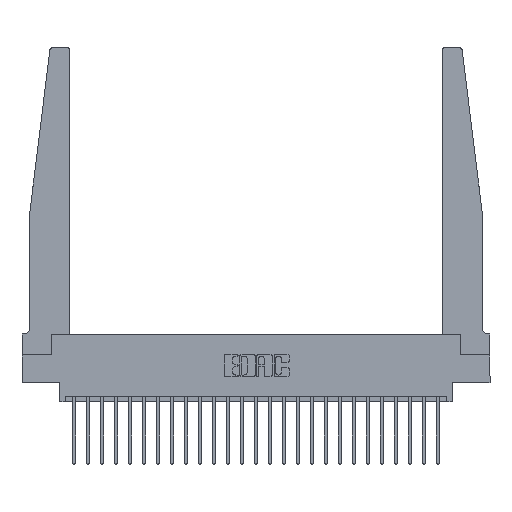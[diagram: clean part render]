
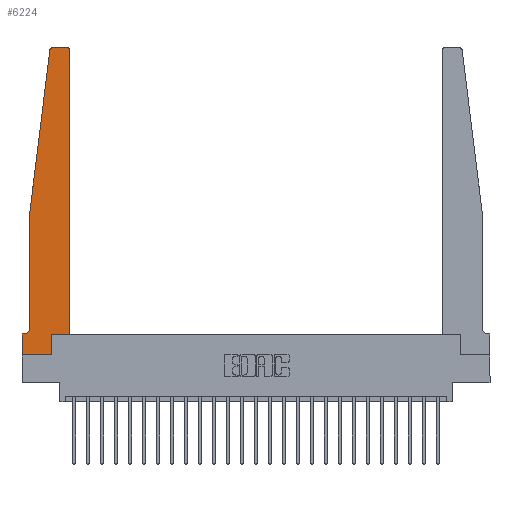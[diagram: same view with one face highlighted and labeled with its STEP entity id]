
A CAD part, top view. The second image highlights one B-rep face of the part: STEP entity #6224.
In plain terms, the highlighted planar face has unit normal (0, 0, 1).
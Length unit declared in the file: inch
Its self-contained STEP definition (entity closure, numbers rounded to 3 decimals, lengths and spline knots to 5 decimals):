
#37 = DIRECTION ( 'NONE',  ( 1., 0., 0. ) ) ;
#206 = CARTESIAN_POINT ( 'NONE',  ( 0., 0., 0.37 ) ) ;
#246 = VERTEX_POINT ( 'NONE', #2233 ) ;
#443 = ORIENTED_EDGE ( 'NONE', *, *, #3222, .T. ) ;
#693 = CARTESIAN_POINT ( 'NONE',  ( 0.015, 0.2375, 0.37 ) ) ;
#827 = VERTEX_POINT ( 'NONE', #11334 ) ;
#934 = CARTESIAN_POINT ( 'NONE',  ( 0.065, 1.25, 0.37 ) ) ;
#1086 = VECTOR ( 'NONE', #23638, 39.37008 ) ;
#1700 = VERTEX_POINT ( 'NONE', #24901 ) ;
#2224 = AXIS2_PLACEMENT_3D ( 'NONE', #3440, #17246, #37 ) ;
#2233 = CARTESIAN_POINT ( 'NONE',  ( 0.425, 0.18, 0.37 ) ) ;
#2616 = CARTESIAN_POINT ( 'NONE',  ( 0.015, 0.1875, 0.37 ) ) ;
#2870 = VERTEX_POINT ( 'NONE', #20106 ) ;
#3074 = LINE ( 'NONE', #10838, #18433 ) ;
#3222 = EDGE_CURVE ( 'NONE', #827, #246, #6039, .T. ) ;
#3346 = CIRCLE ( 'NONE', #17510, 0.03 ) ;
#3440 = CARTESIAN_POINT ( 'NONE',  ( 0., 0.1875, 0.37 ) ) ;
#3684 = FACE_OUTER_BOUND ( 'NONE', #24782, .T. ) ;
#3710 = ORIENTED_EDGE ( 'NONE', *, *, #11147, .T. ) ;
#4295 = LINE ( 'NONE', #21399, #15487 ) ;
#4712 = DIRECTION ( 'NONE',  ( -1., 0., 0. ) ) ;
#5013 = LINE ( 'NONE', #12251, #8605 ) ;
#5020 = EDGE_CURVE ( 'NONE', #12690, #18653, #7843, .T. ) ;
#5141 = ORIENTED_EDGE ( 'NONE', *, *, #5020, .T. ) ;
#5254 = LINE ( 'NONE', #13012, #12823 ) ;
#5432 = AXIS2_PLACEMENT_3D ( 'NONE', #16835, #18852, #17077 ) ;
#5801 = DIRECTION ( 'NONE',  ( 0., -1., 0. ) ) ;
#6039 = LINE ( 'NONE', #19218, #1086 ) ;
#6224 = ADVANCED_FACE ( 'NONE', ( #3684 ), #9534, .T. ) ;
#6436 = CARTESIAN_POINT ( 'NONE',  ( 0., 0., 0.37 ) ) ;
#6754 = DIRECTION ( 'NONE',  ( -0.122, -0.992, 0. ) ) ;
#6797 = CIRCLE ( 'NONE', #20960, 0.05 ) ;
#7299 = DIRECTION ( 'NONE',  ( 0., 1., 0. ) ) ;
#7397 = DIRECTION ( 'NONE',  ( 1., 0., 0. ) ) ;
#7843 = LINE ( 'NONE', #9501, #24765 ) ;
#8056 = LINE ( 'NONE', #8171, #11484 ) ;
#8171 = CARTESIAN_POINT ( 'NONE',  ( 0.065, 0.1875, 0.37 ) ) ;
#8605 = VECTOR ( 'NONE', #24274, 39.37008 ) ;
#9182 = DIRECTION ( 'NONE',  ( 0., 0., 1. ) ) ;
#9501 = CARTESIAN_POINT ( 'NONE',  ( 0.065, 1.25, 0.37 ) ) ;
#9534 = PLANE ( 'NONE',  #2224 ) ;
#9775 = VERTEX_POINT ( 'NONE', #18878 ) ;
#9941 = ORIENTED_EDGE ( 'NONE', *, *, #11010, .T. ) ;
#10058 = EDGE_CURVE ( 'NONE', #12514, #24660, #14566, .T. ) ;
#10298 = EDGE_CURVE ( 'NONE', #15046, #2870, #18387, .T. ) ;
#10838 = CARTESIAN_POINT ( 'NONE',  ( 0.425, 0.18, 0.37 ) ) ;
#10945 = ORIENTED_EDGE ( 'NONE', *, *, #16645, .T. ) ;
#10990 = ORIENTED_EDGE ( 'NONE', *, *, #12450, .T. ) ;
#11010 = EDGE_CURVE ( 'NONE', #9775, #12690, #18284, .T. ) ;
#11147 = EDGE_CURVE ( 'NONE', #246, #15046, #3074, .T. ) ;
#11334 = CARTESIAN_POINT ( 'NONE',  ( 0.2605, 0.18, 0.37 ) ) ;
#11484 = VECTOR ( 'NONE', #12285, 39.37008 ) ;
#12251 = CARTESIAN_POINT ( 'NONE',  ( 0., 0., 0.37 ) ) ;
#12285 = DIRECTION ( 'NONE',  ( -1., 0., 0. ) ) ;
#12450 = EDGE_CURVE ( 'NONE', #19565, #19176, #8056, .T. ) ;
#12497 = ORIENTED_EDGE ( 'NONE', *, *, #16166, .T. ) ;
#12514 = VERTEX_POINT ( 'NONE', #206 ) ;
#12604 = CARTESIAN_POINT ( 'NONE',  ( 0.2605, 0., 0.37 ) ) ;
#12670 = EDGE_CURVE ( 'NONE', #18653, #19565, #6797, .T. ) ;
#12690 = VERTEX_POINT ( 'NONE', #24227 ) ;
#12823 = VECTOR ( 'NONE', #7299, 39.37008 ) ;
#12968 = ORIENTED_EDGE ( 'NONE', *, *, #15779, .T. ) ;
#13012 = CARTESIAN_POINT ( 'NONE',  ( 0.2605, 0.18, 0.37 ) ) ;
#13527 = EDGE_CURVE ( 'NONE', #24660, #827, #5254, .T. ) ;
#13810 = CARTESIAN_POINT ( 'NONE',  ( 0.425, 2.72, 0.37 ) ) ;
#13996 = CARTESIAN_POINT ( 'NONE',  ( 0.065, 0.2375, 0.37 ) ) ;
#14085 = CARTESIAN_POINT ( 'NONE',  ( 0., 0.1875, 0.37 ) ) ;
#14566 = LINE ( 'NONE', #6436, #18272 ) ;
#15046 = VERTEX_POINT ( 'NONE', #13810 ) ;
#15487 = VECTOR ( 'NONE', #17374, 39.37008 ) ;
#15779 = EDGE_CURVE ( 'NONE', #2870, #1700, #4295, .T. ) ;
#16166 = EDGE_CURVE ( 'NONE', #1700, #9775, #3346, .T. ) ;
#16645 = EDGE_CURVE ( 'NONE', #19176, #12514, #5013, .T. ) ;
#16835 = CARTESIAN_POINT ( 'NONE',  ( 0.395, 2.72, 0.37 ) ) ;
#17077 = DIRECTION ( 'NONE',  ( 1., 0., 0. ) ) ;
#17246 = DIRECTION ( 'NONE',  ( 0., 0., 1. ) ) ;
#17374 = DIRECTION ( 'NONE',  ( -1., 0., 0. ) ) ;
#17510 = AXIS2_PLACEMENT_3D ( 'NONE', #22445, #9182, #7397 ) ;
#18272 = VECTOR ( 'NONE', #18471, 39.37008 ) ;
#18284 = LINE ( 'NONE', #934, #23357 ) ;
#18387 = CIRCLE ( 'NONE', #5432, 0.03 ) ;
#18433 = VECTOR ( 'NONE', #22578, 39.37008 ) ;
#18471 = DIRECTION ( 'NONE',  ( 1., 0., 0. ) ) ;
#18653 = VERTEX_POINT ( 'NONE', #13996 ) ;
#18852 = DIRECTION ( 'NONE',  ( 0., 0., 1. ) ) ;
#18878 = CARTESIAN_POINT ( 'NONE',  ( 0.24675, 2.72367, 0.37 ) ) ;
#19176 = VERTEX_POINT ( 'NONE', #14085 ) ;
#19218 = CARTESIAN_POINT ( 'NONE',  ( 0.425, 0.18, 0.37 ) ) ;
#19565 = VERTEX_POINT ( 'NONE', #2616 ) ;
#20106 = CARTESIAN_POINT ( 'NONE',  ( 0.395, 2.75, 0.37 ) ) ;
#20153 = ORIENTED_EDGE ( 'NONE', *, *, #13527, .T. ) ;
#20960 = AXIS2_PLACEMENT_3D ( 'NONE', #693, #22061, #4712 ) ;
#21320 = ORIENTED_EDGE ( 'NONE', *, *, #12670, .T. ) ;
#21399 = CARTESIAN_POINT ( 'NONE',  ( 0.25, 2.75, 0.37 ) ) ;
#22061 = DIRECTION ( 'NONE',  ( 0., 0., -1. ) ) ;
#22445 = CARTESIAN_POINT ( 'NONE',  ( 0.27653, 2.72, 0.37 ) ) ;
#22578 = DIRECTION ( 'NONE',  ( 0., 1., 0. ) ) ;
#22616 = ORIENTED_EDGE ( 'NONE', *, *, #10058, .T. ) ;
#23357 = VECTOR ( 'NONE', #6754, 39.37008 ) ;
#23638 = DIRECTION ( 'NONE',  ( 1., 0., 0. ) ) ;
#23773 = ORIENTED_EDGE ( 'NONE', *, *, #10298, .T. ) ;
#24227 = CARTESIAN_POINT ( 'NONE',  ( 0.065, 1.25, 0.37 ) ) ;
#24274 = DIRECTION ( 'NONE',  ( 0., -1., 0. ) ) ;
#24660 = VERTEX_POINT ( 'NONE', #12604 ) ;
#24765 = VECTOR ( 'NONE', #5801, 39.37008 ) ;
#24782 = EDGE_LOOP ( 'NONE', ( #12968, #12497, #9941, #5141, #21320, #10990, #10945, #22616, #20153, #443, #3710, #23773 ) ) ;
#24901 = CARTESIAN_POINT ( 'NONE',  ( 0.27653, 2.75, 0.37 ) ) ;
